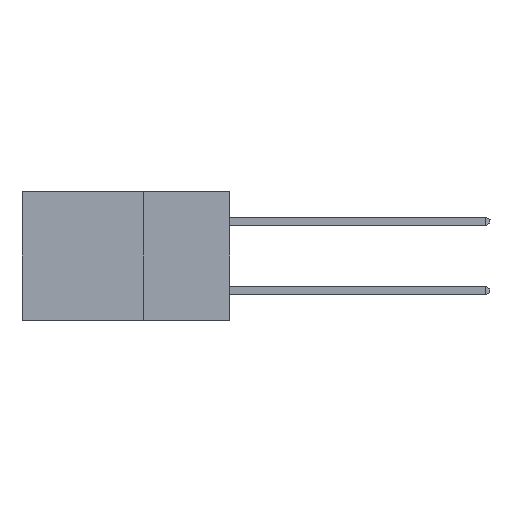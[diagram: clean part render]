
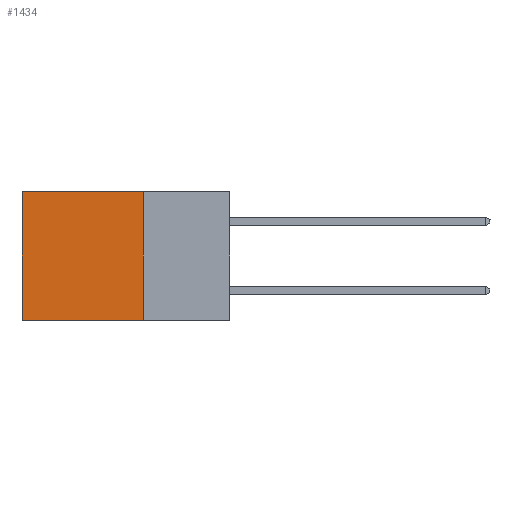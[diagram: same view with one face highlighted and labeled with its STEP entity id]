
A CAD part, left-side view. The second image highlights one B-rep face of the part: STEP entity #1434.
In plain terms, the highlighted planar face has unit normal (-1, 0, 0).
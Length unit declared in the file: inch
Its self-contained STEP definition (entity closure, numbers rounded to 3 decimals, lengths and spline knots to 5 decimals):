
#413 = VERTEX_POINT ( 'NONE', #3239 ) ;
#806 = EDGE_CURVE ( 'NONE', #25614, #14349, #7404, .T. ) ;
#1434 = ADVANCED_FACE ( 'NONE', ( #14906 ), #5202, .F. ) ;
#1910 = CARTESIAN_POINT ( 'NONE',  ( 0.298, 0.25, 0. ) ) ;
#3239 = CARTESIAN_POINT ( 'NONE',  ( 0.298, 0.6, 0. ) ) ;
#3315 = EDGE_CURVE ( 'NONE', #413, #14349, #23206, .T. ) ;
#3538 = CARTESIAN_POINT ( 'NONE',  ( 0.298, 0.25, 0. ) ) ;
#5160 = CARTESIAN_POINT ( 'NONE',  ( 0.298, 0.25, 0. ) ) ;
#5202 = PLANE ( 'NONE',  #27336 ) ;
#5401 = DIRECTION ( 'NONE',  ( 0., 0., -1. ) ) ;
#5657 = VECTOR ( 'NONE', #22171, 39.37008 ) ;
#6350 = EDGE_CURVE ( 'NONE', #20982, #413, #12076, .T. ) ;
#7192 = CARTESIAN_POINT ( 'NONE',  ( 0.298, 0.6, -0.37 ) ) ;
#7404 = LINE ( 'NONE', #26578, #22922 ) ;
#7830 = ORIENTED_EDGE ( 'NONE', *, *, #6350, .T. ) ;
#8756 = ORIENTED_EDGE ( 'NONE', *, *, #14171, .F. ) ;
#9405 = DIRECTION ( 'NONE',  ( 0., 1., 0. ) ) ;
#9924 = DIRECTION ( 'NONE',  ( 1., 0., 0. ) ) ;
#10776 = DIRECTION ( 'NONE',  ( 0., 0., -1. ) ) ;
#11110 = LINE ( 'NONE', #3538, #22066 ) ;
#12076 = LINE ( 'NONE', #5160, #5657 ) ;
#14171 = EDGE_CURVE ( 'NONE', #20982, #25614, #11110, .T. ) ;
#14349 = VERTEX_POINT ( 'NONE', #7192 ) ;
#14906 = FACE_OUTER_BOUND ( 'NONE', #23172, .T. ) ;
#14968 = CARTESIAN_POINT ( 'NONE',  ( 0.298, 0.25, -0.37 ) ) ;
#15108 = ORIENTED_EDGE ( 'NONE', *, *, #3315, .T. ) ;
#16749 = VECTOR ( 'NONE', #10776, 39.37008 ) ;
#19569 = CARTESIAN_POINT ( 'NONE',  ( 0.298, 0.25, 0. ) ) ;
#20452 = DIRECTION ( 'NONE',  ( 0., 0., -1. ) ) ;
#20982 = VERTEX_POINT ( 'NONE', #1910 ) ;
#22066 = VECTOR ( 'NONE', #20452, 39.37008 ) ;
#22171 = DIRECTION ( 'NONE',  ( 0., 1., 0. ) ) ;
#22922 = VECTOR ( 'NONE', #9405, 39.37008 ) ;
#23172 = EDGE_LOOP ( 'NONE', ( #15108, #28880, #8756, #7830 ) ) ;
#23206 = LINE ( 'NONE', #27816, #16749 ) ;
#25614 = VERTEX_POINT ( 'NONE', #14968 ) ;
#26578 = CARTESIAN_POINT ( 'NONE',  ( 0.298, 0.25, -0.37 ) ) ;
#27336 = AXIS2_PLACEMENT_3D ( 'NONE', #19569, #9924, #5401 ) ;
#27816 = CARTESIAN_POINT ( 'NONE',  ( 0.298, 0.6, 0. ) ) ;
#28880 = ORIENTED_EDGE ( 'NONE', *, *, #806, .F. ) ;
